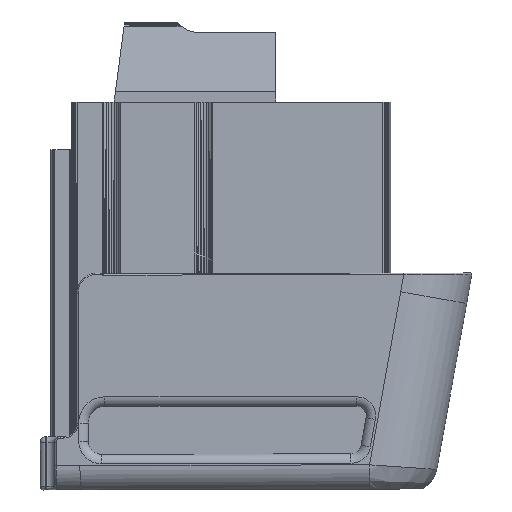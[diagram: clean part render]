
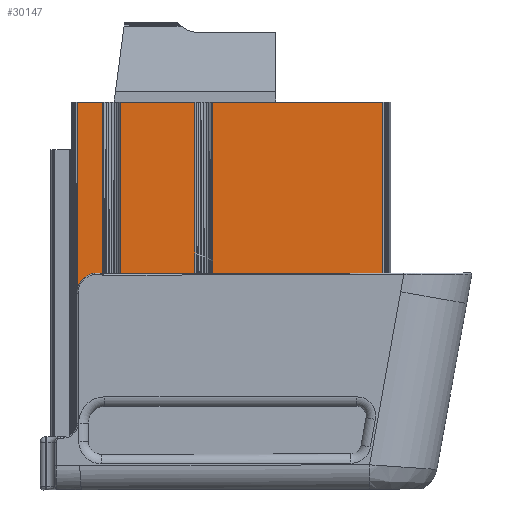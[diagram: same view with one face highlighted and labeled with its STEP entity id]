
A CAD part, left-side view. The second image highlights one B-rep face of the part: STEP entity #30147.
In plain terms, the highlighted planar face has unit normal (-1, 0, 0).
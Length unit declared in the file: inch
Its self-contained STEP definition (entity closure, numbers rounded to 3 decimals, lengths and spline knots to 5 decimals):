
#188=CIRCLE('',#32182,0.15);
#615=FACE_OUTER_BOUND('',#2826,.T.);
#2826=EDGE_LOOP('',(#21070,#21071,#21072,#21073,#21074,#21075,#21076,#21077,
#21078,#21079,#21080,#21081,#21082));
#5144=LINE('',#44580,#9237);
#5270=LINE('',#44962,#9363);
#5293=LINE('',#45009,#9386);
#5855=LINE('',#46136,#9948);
#5856=LINE('',#46138,#9949);
#5857=LINE('',#46140,#9950);
#5858=LINE('',#46142,#9951);
#5859=LINE('',#46143,#9952);
#5860=LINE('',#46145,#9953);
#5861=LINE('',#46147,#9954);
#5862=LINE('',#46148,#9955);
#5863=LINE('',#46149,#9956);
#9237=VECTOR('',#35200,0.3937);
#9363=VECTOR('',#35440,0.3937);
#9386=VECTOR('',#35481,0.3937);
#9948=VECTOR('',#36389,0.3937);
#9949=VECTOR('',#36390,0.3937);
#9950=VECTOR('',#36391,0.3937);
#9951=VECTOR('',#36392,0.3937);
#9952=VECTOR('',#36393,0.3937);
#9953=VECTOR('',#36394,0.3937);
#9954=VECTOR('',#36395,0.3937);
#9955=VECTOR('',#36396,0.3937);
#9956=VECTOR('',#36397,0.3937);
#13233=VERTEX_POINT('',#44147);
#13234=VERTEX_POINT('',#44149);
#13328=VERTEX_POINT('',#44578);
#13415=VERTEX_POINT('',#44958);
#13417=VERTEX_POINT('',#44961);
#13430=VERTEX_POINT('',#45005);
#13432=VERTEX_POINT('',#45008);
#13824=VERTEX_POINT('',#46135);
#13825=VERTEX_POINT('',#46137);
#13826=VERTEX_POINT('',#46139);
#13827=VERTEX_POINT('',#46141);
#13828=VERTEX_POINT('',#46144);
#13829=VERTEX_POINT('',#46146);
#15370=EDGE_CURVE('',#13234,#13233,#188,.T.);
#15487=EDGE_CURVE('',#13233,#13328,#5144,.T.);
#15624=EDGE_CURVE('',#13417,#13415,#5270,.T.);
#15647=EDGE_CURVE('',#13432,#13430,#5293,.T.);
#16210=EDGE_CURVE('',#13234,#13824,#5855,.T.);
#16211=EDGE_CURVE('',#13328,#13825,#5856,.T.);
#16212=EDGE_CURVE('',#13826,#13825,#5857,.T.);
#16213=EDGE_CURVE('',#13827,#13826,#5858,.T.);
#16214=EDGE_CURVE('',#13827,#13432,#5859,.T.);
#16215=EDGE_CURVE('',#13828,#13430,#5860,.T.);
#16216=EDGE_CURVE('',#13829,#13828,#5861,.T.);
#16217=EDGE_CURVE('',#13829,#13417,#5862,.T.);
#16218=EDGE_CURVE('',#13824,#13415,#5863,.T.);
#21070=ORIENTED_EDGE('',*,*,#16210,.F.);
#21071=ORIENTED_EDGE('',*,*,#15370,.T.);
#21072=ORIENTED_EDGE('',*,*,#15487,.T.);
#21073=ORIENTED_EDGE('',*,*,#16211,.T.);
#21074=ORIENTED_EDGE('',*,*,#16212,.F.);
#21075=ORIENTED_EDGE('',*,*,#16213,.F.);
#21076=ORIENTED_EDGE('',*,*,#16214,.T.);
#21077=ORIENTED_EDGE('',*,*,#15647,.T.);
#21078=ORIENTED_EDGE('',*,*,#16215,.F.);
#21079=ORIENTED_EDGE('',*,*,#16216,.F.);
#21080=ORIENTED_EDGE('',*,*,#16217,.T.);
#21081=ORIENTED_EDGE('',*,*,#15624,.T.);
#21082=ORIENTED_EDGE('',*,*,#16218,.F.);
#27972=PLANE('',#32462);
#30147=ADVANCED_FACE('',(#615),#27972,.T.);
#32182=AXIS2_PLACEMENT_3D('',#44150,#35032,#35033);
#32462=AXIS2_PLACEMENT_3D('',#46134,#36387,#36388);
#35032=DIRECTION('center_axis',(1.,0.,0.));
#35033=DIRECTION('ref_axis',(0.,0.,1.));
#35200=DIRECTION('',(0.,-1.,0.003));
#35440=DIRECTION('',(0.,0.,1.));
#35481=DIRECTION('',(0.,0.,1.));
#36387=DIRECTION('center_axis',(-1.,0.,0.));
#36388=DIRECTION('ref_axis',(0.,-1.,0.003));
#36389=DIRECTION('',(0.,0.,1.));
#36390=DIRECTION('',(0.,0.,1.));
#36391=DIRECTION('',(0.,-1.,0.));
#36392=DIRECTION('',(0.,0.,1.));
#36393=DIRECTION('',(0.,1.,-0.003));
#36394=DIRECTION('',(0.,-1.,0.));
#36395=DIRECTION('',(0.,0.,1.));
#36396=DIRECTION('',(0.,1.,-0.003));
#36397=DIRECTION('',(0.,-1.,0.));
#44147=CARTESIAN_POINT('',(-0.42541,-2.36167,-3.25323));
#44149=CARTESIAN_POINT('',(-0.42541,-2.16807,-3.37653));
#44150=CARTESIAN_POINT('Origin',(-0.42541,-2.31675,-3.39634));
#44578=CARTESIAN_POINT('',(-0.42541,-4.45158,-3.24735));
#44580=CARTESIAN_POINT('',(-0.42541,-3.09088,-3.25118));
#44958=CARTESIAN_POINT('',(-0.42541,-2.35578,-1.96997));
#44961=CARTESIAN_POINT('',(-0.42541,-2.35578,-3.24846));
#44962=CARTESIAN_POINT('',(-0.42541,-2.35578,-6.86969));
#45005=CARTESIAN_POINT('',(-0.42541,-3.04476,-1.96997));
#45008=CARTESIAN_POINT('',(-0.42541,-3.04476,-3.24652));
#45009=CARTESIAN_POINT('',(-0.42541,-3.04476,-6.76057));
#46134=CARTESIAN_POINT('Origin',(-0.42541,-3.88067,-4.87912));
#46135=CARTESIAN_POINT('',(-0.42541,-2.16807,-1.96997));
#46136=CARTESIAN_POINT('',(-0.42541,-2.16807,-6.89942));
#46137=CARTESIAN_POINT('',(-0.42541,-4.45158,-1.96997));
#46138=CARTESIAN_POINT('',(-0.42541,-4.45158,-6.53775));
#46139=CARTESIAN_POINT('',(-0.42541,-3.18114,-1.96997));
#46140=CARTESIAN_POINT('',(-0.42541,-3.18114,-1.96997));
#46141=CARTESIAN_POINT('',(-0.42541,-3.18114,-3.24614));
#46142=CARTESIAN_POINT('',(-0.42541,-3.18114,-6.73896));
#46143=CARTESIAN_POINT('',(-0.42541,-3.51479,-3.2452));
#46144=CARTESIAN_POINT('',(-0.42541,-2.49217,-1.96997));
#46145=CARTESIAN_POINT('',(-0.42541,-2.49217,-1.96997));
#46146=CARTESIAN_POINT('',(-0.42541,-2.49217,-3.24807));
#46147=CARTESIAN_POINT('',(-0.42541,-2.49217,-6.84809));
#46148=CARTESIAN_POINT('',(-0.42541,-3.51479,-3.2452));
#46149=CARTESIAN_POINT('',(-0.42541,-2.16807,-1.96997));
